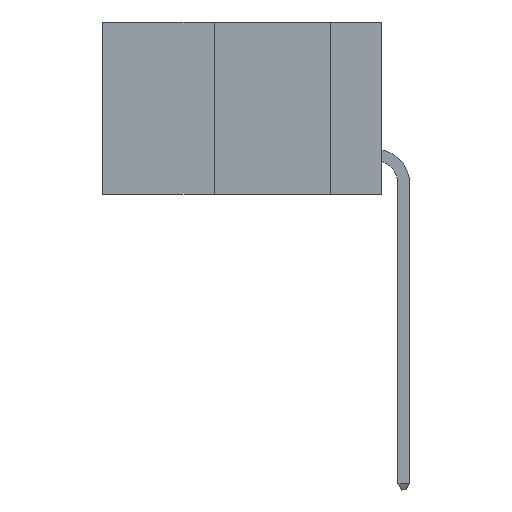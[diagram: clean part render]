
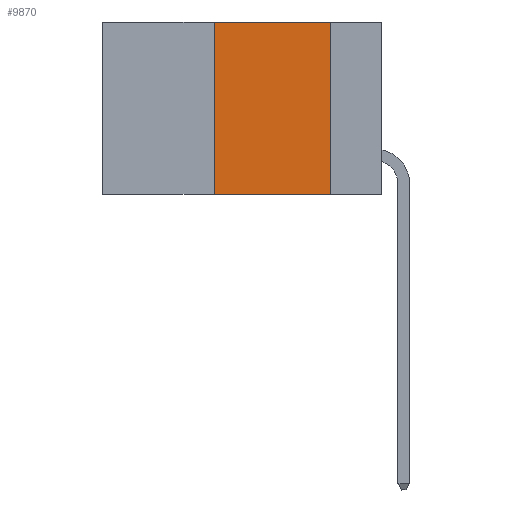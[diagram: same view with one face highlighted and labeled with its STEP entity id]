
A CAD part, left-side view. The second image highlights one B-rep face of the part: STEP entity #9870.
In plain terms, the highlighted planar face has unit normal (-1, 0, 0).
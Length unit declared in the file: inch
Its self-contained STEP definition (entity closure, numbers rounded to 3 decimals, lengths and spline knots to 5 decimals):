
#304 = CARTESIAN_POINT ( 'NONE',  ( 0., 0.36, 0. ) ) ;
#2781 = FACE_OUTER_BOUND ( 'NONE', #14145, .T. ) ;
#2901 = DIRECTION ( 'NONE',  ( 0., -1., 0. ) ) ;
#3251 = CARTESIAN_POINT ( 'NONE',  ( 0., 0.11, 0. ) ) ;
#3457 = VERTEX_POINT ( 'NONE', #11867 ) ;
#4595 = LINE ( 'NONE', #15272, #15671 ) ;
#5138 = CARTESIAN_POINT ( 'NONE',  ( 0., 0.11, 0. ) ) ;
#6087 = LINE ( 'NONE', #19776, #24765 ) ;
#6270 = LINE ( 'NONE', #3251, #15761 ) ;
#7268 = AXIS2_PLACEMENT_3D ( 'NONE', #16298, #14427, #20541 ) ;
#7684 = ORIENTED_EDGE ( 'NONE', *, *, #25733, .F. ) ;
#8267 = VERTEX_POINT ( 'NONE', #5138 ) ;
#8984 = VERTEX_POINT ( 'NONE', #18225 ) ;
#9870 = ADVANCED_FACE ( 'NONE', ( #2781 ), #19413, .F. ) ;
#10561 = CARTESIAN_POINT ( 'NONE',  ( 0., 0.11, -0.37 ) ) ;
#11867 = CARTESIAN_POINT ( 'NONE',  ( 0., 0.36, 0. ) ) ;
#12180 = ORIENTED_EDGE ( 'NONE', *, *, #21152, .F. ) ;
#13000 = VERTEX_POINT ( 'NONE', #10561 ) ;
#13182 = ORIENTED_EDGE ( 'NONE', *, *, #15743, .F. ) ;
#14145 = EDGE_LOOP ( 'NONE', ( #7684, #13182, #12180, #21369 ) ) ;
#14427 = DIRECTION ( 'NONE',  ( 1., 0., 0. ) ) ;
#15272 = CARTESIAN_POINT ( 'NONE',  ( 0., 0.6, -0.37 ) ) ;
#15671 = VECTOR ( 'NONE', #2901, 39.37008 ) ;
#15743 = EDGE_CURVE ( 'NONE', #3457, #8267, #6087, .T. ) ;
#15761 = VECTOR ( 'NONE', #23493, 39.37008 ) ;
#16298 = CARTESIAN_POINT ( 'NONE',  ( 0., 0.6, 0. ) ) ;
#17590 = EDGE_CURVE ( 'NONE', #8984, #13000, #4595, .T. ) ;
#18225 = CARTESIAN_POINT ( 'NONE',  ( 0., 0.36, -0.37 ) ) ;
#19413 = PLANE ( 'NONE',  #7268 ) ;
#19776 = CARTESIAN_POINT ( 'NONE',  ( 0., 0.6, 0. ) ) ;
#20541 = DIRECTION ( 'NONE',  ( 0., 0., -1. ) ) ;
#20728 = DIRECTION ( 'NONE',  ( 0., 0., 1. ) ) ;
#21152 = EDGE_CURVE ( 'NONE', #8984, #3457, #22750, .T. ) ;
#21369 = ORIENTED_EDGE ( 'NONE', *, *, #17590, .T. ) ;
#21481 = VECTOR ( 'NONE', #20728, 39.37008 ) ;
#22750 = LINE ( 'NONE', #304, #21481 ) ;
#23493 = DIRECTION ( 'NONE',  ( 0., 0., -1. ) ) ;
#23597 = DIRECTION ( 'NONE',  ( 0., -1., 0. ) ) ;
#24765 = VECTOR ( 'NONE', #23597, 39.37008 ) ;
#25733 = EDGE_CURVE ( 'NONE', #8267, #13000, #6270, .T. ) ;
